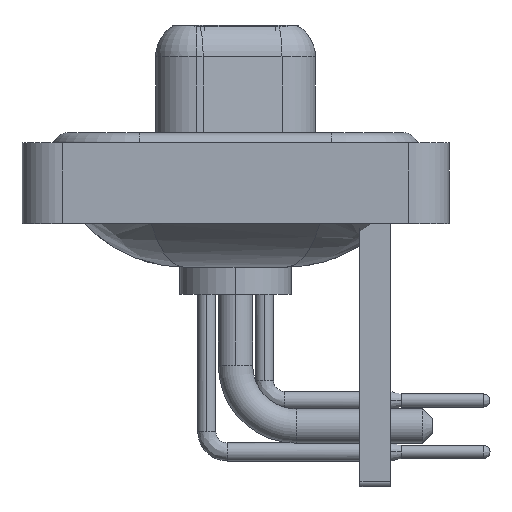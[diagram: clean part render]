
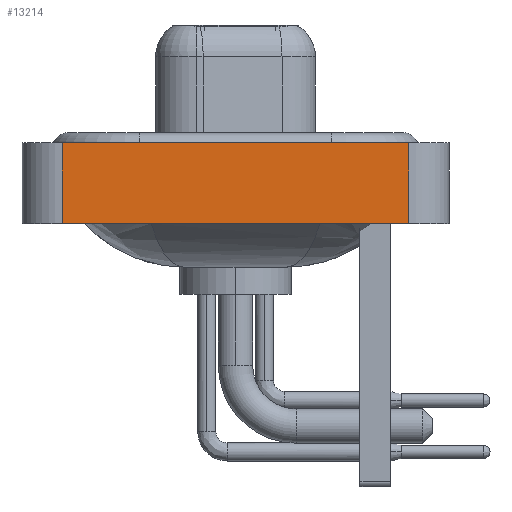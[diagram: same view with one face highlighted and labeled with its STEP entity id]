
A CAD part, left-side view. The second image highlights one B-rep face of the part: STEP entity #13214.
In plain terms, the highlighted planar face has unit normal (-1, 0, 0).
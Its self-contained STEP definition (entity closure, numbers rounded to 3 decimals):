
#617 = DIRECTION ( 'NONE',  ( 0., -1., 0. ) ) ;
#1240 = ORIENTED_EDGE ( 'NONE', *, *, #17602, .F. ) ;
#1705 = FACE_OUTER_BOUND ( 'NONE', #2864, .T. ) ;
#2089 = VERTEX_POINT ( 'NONE', #16119 ) ;
#2322 = CARTESIAN_POINT ( 'NONE',  ( -7.35, -8.55, 0.4 ) ) ;
#2346 = LINE ( 'NONE', #20014, #6740 ) ;
#2864 = EDGE_LOOP ( 'NONE', ( #12854, #21151, #1240, #19335 ) ) ;
#5262 = VERTEX_POINT ( 'NONE', #2322 ) ;
#5854 = VECTOR ( 'NONE', #617, 1000. ) ;
#6100 = CARTESIAN_POINT ( 'NONE',  ( -7.35, 8.55, -3.6 ) ) ;
#6740 = VECTOR ( 'NONE', #21081, 1000. ) ;
#6815 = LINE ( 'NONE', #24534, #16930 ) ;
#7330 = CARTESIAN_POINT ( 'NONE',  ( -7.35, -8.55, -3.6 ) ) ;
#9543 = DIRECTION ( 'NONE',  ( -1., 0., 0. ) ) ;
#10028 = LINE ( 'NONE', #19482, #23104 ) ;
#11190 = PLANE ( 'NONE',  #16036 ) ;
#12424 = LINE ( 'NONE', #18065, #5854 ) ;
#12854 = ORIENTED_EDGE ( 'NONE', *, *, #21178, .T. ) ;
#13214 = ADVANCED_FACE ( 'NONE', ( #1705 ), #11190, .T. ) ;
#15648 = DIRECTION ( 'NONE',  ( 0., 0., 1. ) ) ;
#15716 = EDGE_CURVE ( 'NONE', #22450, #24597, #6815, .T. ) ;
#16036 = AXIS2_PLACEMENT_3D ( 'NONE', #7330, #9543, #22980 ) ;
#16119 = CARTESIAN_POINT ( 'NONE',  ( -7.35, 8.55, 0.4 ) ) ;
#16298 = CARTESIAN_POINT ( 'NONE',  ( -7.35, -8.55, -3.6 ) ) ;
#16930 = VECTOR ( 'NONE', #23680, 1000. ) ;
#17602 = EDGE_CURVE ( 'NONE', #22450, #2089, #10028, .T. ) ;
#18065 = CARTESIAN_POINT ( 'NONE',  ( -7.35, -8.55, 0.4 ) ) ;
#19335 = ORIENTED_EDGE ( 'NONE', *, *, #15716, .T. ) ;
#19482 = CARTESIAN_POINT ( 'NONE',  ( -7.35, 8.55, -3.6 ) ) ;
#20014 = CARTESIAN_POINT ( 'NONE',  ( -7.35, -8.55, -3.6 ) ) ;
#21081 = DIRECTION ( 'NONE',  ( 0., 0., 1. ) ) ;
#21151 = ORIENTED_EDGE ( 'NONE', *, *, #25018, .F. ) ;
#21178 = EDGE_CURVE ( 'NONE', #24597, #5262, #2346, .T. ) ;
#22450 = VERTEX_POINT ( 'NONE', #6100 ) ;
#22980 = DIRECTION ( 'NONE',  ( 0., 0., 1. ) ) ;
#23104 = VECTOR ( 'NONE', #15648, 1000. ) ;
#23680 = DIRECTION ( 'NONE',  ( 0., -1., 0. ) ) ;
#24534 = CARTESIAN_POINT ( 'NONE',  ( -7.35, -8.55, -3.6 ) ) ;
#24597 = VERTEX_POINT ( 'NONE', #16298 ) ;
#25018 = EDGE_CURVE ( 'NONE', #2089, #5262, #12424, .T. ) ;
